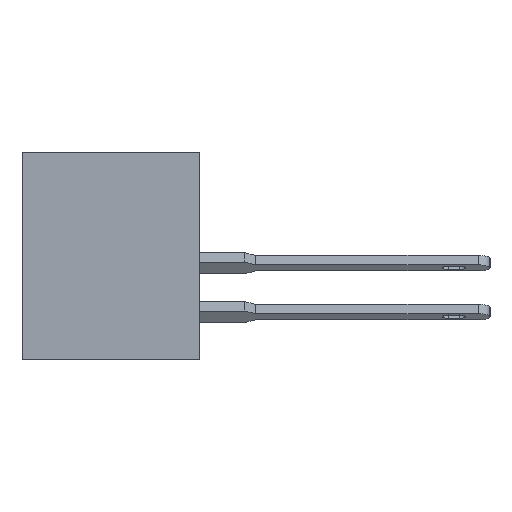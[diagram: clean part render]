
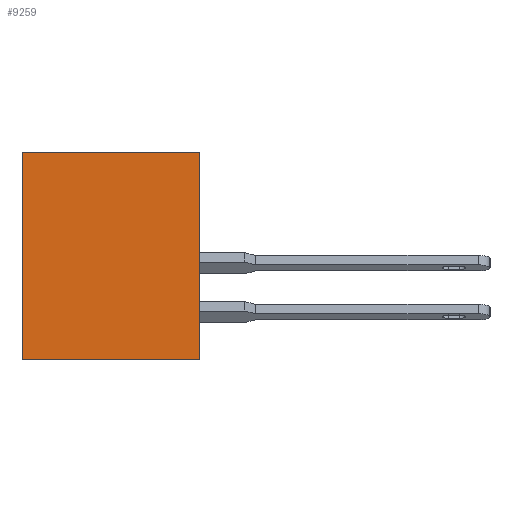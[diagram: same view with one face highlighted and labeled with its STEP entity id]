
A CAD part, left-side view. The second image highlights one B-rep face of the part: STEP entity #9259.
In plain terms, the highlighted planar face has unit normal (-1, 0, 0).
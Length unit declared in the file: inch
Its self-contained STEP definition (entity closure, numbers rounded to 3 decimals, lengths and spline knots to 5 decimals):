
#226 = ORIENTED_EDGE ( 'NONE', *, *, #14848, .F. ) ;
#1884 = LINE ( 'NONE', #5155, #5338 ) ;
#2459 = CARTESIAN_POINT ( 'NONE',  ( 0., 0., 0. ) ) ;
#2762 = CARTESIAN_POINT ( 'NONE',  ( 0., 0.453, 0. ) ) ;
#3473 = VERTEX_POINT ( 'NONE', #6562 ) ;
#3494 = VERTEX_POINT ( 'NONE', #2762 ) ;
#4165 = CARTESIAN_POINT ( 'NONE',  ( 0., 0.453, 0. ) ) ;
#5075 = EDGE_CURVE ( 'NONE', #3473, #11309, #13714, .T. ) ;
#5155 = CARTESIAN_POINT ( 'NONE',  ( 0., 0.453, 0. ) ) ;
#5243 = VECTOR ( 'NONE', #14146, 39.37008 ) ;
#5338 = VECTOR ( 'NONE', #7550, 39.37008 ) ;
#5373 = CARTESIAN_POINT ( 'NONE',  ( 0., 0., 0. ) ) ;
#6562 = CARTESIAN_POINT ( 'NONE',  ( 0., 0., -0.531 ) ) ;
#6635 = VECTOR ( 'NONE', #6638, 39.37008 ) ;
#6638 = DIRECTION ( 'NONE',  ( 0., 0., 1. ) ) ;
#7550 = DIRECTION ( 'NONE',  ( 0., -1., 0. ) ) ;
#7802 = EDGE_CURVE ( 'NONE', #15606, #3473, #13456, .T. ) ;
#8902 = LINE ( 'NONE', #12778, #6635 ) ;
#8948 = PLANE ( 'NONE',  #13162 ) ;
#9259 = ADVANCED_FACE ( 'NONE', ( #14749 ), #8948, .F. ) ;
#9518 = VECTOR ( 'NONE', #13959, 39.37008 ) ;
#9884 = EDGE_LOOP ( 'NONE', ( #15057, #226, #10943, #13598 ) ) ;
#10943 = ORIENTED_EDGE ( 'NONE', *, *, #15579, .F. ) ;
#11309 = VERTEX_POINT ( 'NONE', #2459 ) ;
#11420 = DIRECTION ( 'NONE',  ( 1., 0., 0. ) ) ;
#11562 = CARTESIAN_POINT ( 'NONE',  ( 0., 0.453, -0.531 ) ) ;
#11697 = CARTESIAN_POINT ( 'NONE',  ( 0., 0.453, -0.531 ) ) ;
#12574 = DIRECTION ( 'NONE',  ( 0., 0., -1. ) ) ;
#12778 = CARTESIAN_POINT ( 'NONE',  ( 0., 0.453, 0. ) ) ;
#13162 = AXIS2_PLACEMENT_3D ( 'NONE', #4165, #11420, #12574 ) ;
#13456 = LINE ( 'NONE', #11697, #5243 ) ;
#13598 = ORIENTED_EDGE ( 'NONE', *, *, #7802, .T. ) ;
#13714 = LINE ( 'NONE', #5373, #9518 ) ;
#13959 = DIRECTION ( 'NONE',  ( 0., 0., 1. ) ) ;
#14146 = DIRECTION ( 'NONE',  ( 0., -1., 0. ) ) ;
#14749 = FACE_OUTER_BOUND ( 'NONE', #9884, .T. ) ;
#14848 = EDGE_CURVE ( 'NONE', #3494, #11309, #1884, .T. ) ;
#15057 = ORIENTED_EDGE ( 'NONE', *, *, #5075, .T. ) ;
#15579 = EDGE_CURVE ( 'NONE', #15606, #3494, #8902, .T. ) ;
#15606 = VERTEX_POINT ( 'NONE', #11562 ) ;
